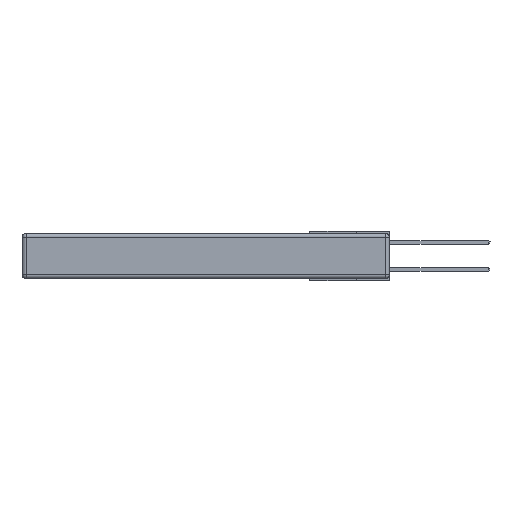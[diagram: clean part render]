
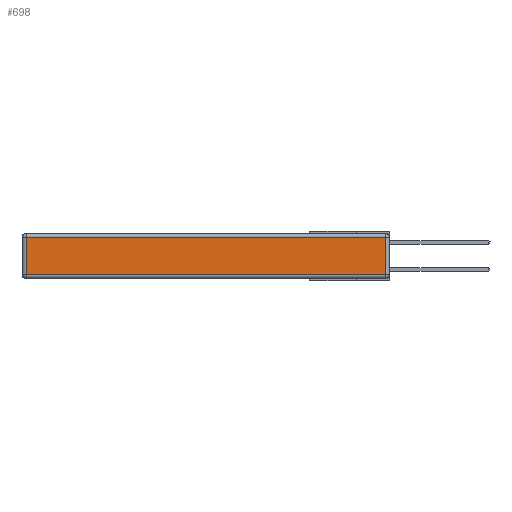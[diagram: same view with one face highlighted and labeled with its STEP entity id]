
A CAD part, left-side view. The second image highlights one B-rep face of the part: STEP entity #698.
In plain terms, the highlighted planar face has unit normal (-1, 0, 0).
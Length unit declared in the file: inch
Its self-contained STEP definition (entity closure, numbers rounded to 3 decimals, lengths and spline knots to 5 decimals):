
#698 = ADVANCED_FACE ( 'NONE', ( #10617 ), #22641, .T. ) ;
#4255 = EDGE_CURVE ( 'NONE', #23139, #20474, #20410, .T. ) ;
#4620 = LINE ( 'NONE', #22049, #6164 ) ;
#6073 = CARTESIAN_POINT ( 'NONE',  ( 0., 2.72, -0.343 ) ) ;
#6164 = VECTOR ( 'NONE', #19861, 39.37008 ) ;
#6791 = LINE ( 'NONE', #23842, #13098 ) ;
#7027 = CARTESIAN_POINT ( 'NONE',  ( 0., 0.03, -0.343 ) ) ;
#7750 = CARTESIAN_POINT ( 'NONE',  ( 0., 0., -0.343 ) ) ;
#8248 = EDGE_CURVE ( 'NONE', #20474, #15987, #4620, .T. ) ;
#9118 = CARTESIAN_POINT ( 'NONE',  ( 0., 0.03, -0.03 ) ) ;
#9397 = CARTESIAN_POINT ( 'NONE',  ( 0., 0.03, -0.313 ) ) ;
#9665 = ORIENTED_EDGE ( 'NONE', *, *, #4255, .T. ) ;
#9984 = CARTESIAN_POINT ( 'NONE',  ( 0., 2.72, -0.03 ) ) ;
#10617 = FACE_OUTER_BOUND ( 'NONE', #10998, .T. ) ;
#10998 = EDGE_LOOP ( 'NONE', ( #19898, #22867, #15860, #9665 ) ) ;
#12896 = DIRECTION ( 'NONE',  ( 0., 0., 1. ) ) ;
#13098 = VECTOR ( 'NONE', #21214, 39.37008 ) ;
#13165 = VECTOR ( 'NONE', #21885, 39.37008 ) ;
#15860 = ORIENTED_EDGE ( 'NONE', *, *, #25562, .T. ) ;
#15987 = VERTEX_POINT ( 'NONE', #9397 ) ;
#18141 = DIRECTION ( 'NONE',  ( 0., 0., -1. ) ) ;
#18631 = CARTESIAN_POINT ( 'NONE',  ( 0., 2.72, -0.313 ) ) ;
#19861 = DIRECTION ( 'NONE',  ( 0., -1., 0. ) ) ;
#19898 = ORIENTED_EDGE ( 'NONE', *, *, #8248, .T. ) ;
#20410 = LINE ( 'NONE', #6073, #28900 ) ;
#20474 = VERTEX_POINT ( 'NONE', #18631 ) ;
#21214 = DIRECTION ( 'NONE',  ( 0., 1., 0. ) ) ;
#21885 = DIRECTION ( 'NONE',  ( 0., 0., 1. ) ) ;
#22049 = CARTESIAN_POINT ( 'NONE',  ( 0., 0., -0.313 ) ) ;
#22641 = PLANE ( 'NONE',  #30729 ) ;
#22867 = ORIENTED_EDGE ( 'NONE', *, *, #29664, .T. ) ;
#23139 = VERTEX_POINT ( 'NONE', #9984 ) ;
#23842 = CARTESIAN_POINT ( 'NONE',  ( 0., 2.75, -0.03 ) ) ;
#25562 = EDGE_CURVE ( 'NONE', #31111, #23139, #6791, .T. ) ;
#26352 = LINE ( 'NONE', #7027, #13165 ) ;
#27752 = DIRECTION ( 'NONE',  ( -1., 0., 0. ) ) ;
#28900 = VECTOR ( 'NONE', #18141, 39.37008 ) ;
#29664 = EDGE_CURVE ( 'NONE', #15987, #31111, #26352, .T. ) ;
#30729 = AXIS2_PLACEMENT_3D ( 'NONE', #7750, #27752, #12896 ) ;
#31111 = VERTEX_POINT ( 'NONE', #9118 ) ;
